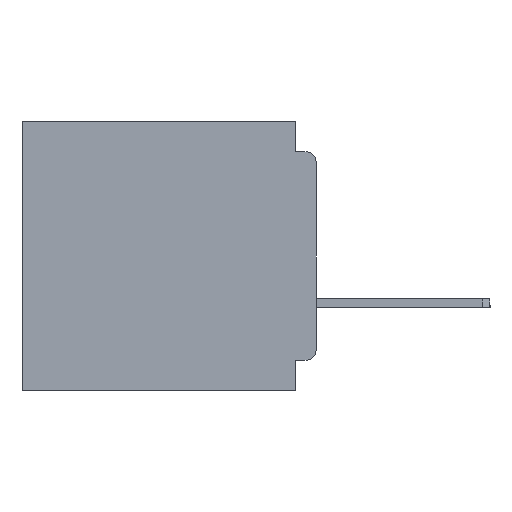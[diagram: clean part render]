
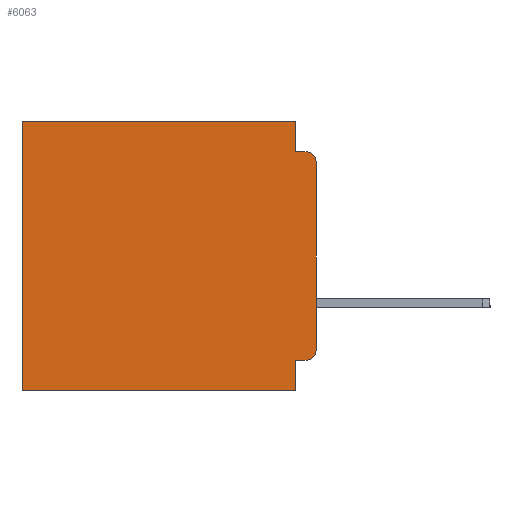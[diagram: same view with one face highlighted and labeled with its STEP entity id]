
A CAD part, left-side view. The second image highlights one B-rep face of the part: STEP entity #6063.
In plain terms, the highlighted planar face has unit normal (-1, 0, 0).
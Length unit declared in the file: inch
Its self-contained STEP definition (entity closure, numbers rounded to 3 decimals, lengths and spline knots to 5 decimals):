
#870 = CARTESIAN_POINT ( 'NONE',  ( 0.3, 0.031, -0.355 ) ) ;
#1079 = DIRECTION ( 'NONE',  ( 0., 0., -1. ) ) ;
#2589 = CARTESIAN_POINT ( 'NONE',  ( 0.3, 0.437, -0.4 ) ) ;
#3789 = VECTOR ( 'NONE', #7308, 39.37008 ) ;
#5596 = ORIENTED_EDGE ( 'NONE', *, *, #23079, .F. ) ;
#6063 = ADVANCED_FACE ( 'NONE', ( #39883 ), #53114, .F. ) ;
#6574 = VERTEX_POINT ( 'NONE', #17588 ) ;
#6836 = EDGE_LOOP ( 'NONE', ( #43528, #13128, #16899, #50039, #42352, #41228, #26954, #5596, #57168, #17152 ) ) ;
#7308 = DIRECTION ( 'NONE',  ( 0., -1., 0. ) ) ;
#7414 = CARTESIAN_POINT ( 'NONE',  ( 0.3, 0.031, 0. ) ) ;
#7686 = VECTOR ( 'NONE', #46446, 39.37008 ) ;
#8356 = EDGE_CURVE ( 'NONE', #29767, #29869, #30248, .T. ) ;
#10212 = CARTESIAN_POINT ( 'NONE',  ( 0.3, 0., 0. ) ) ;
#12451 = LINE ( 'NONE', #47709, #46542 ) ;
#12472 = CIRCLE ( 'NONE', #53079, 0.015 ) ;
#12743 = LINE ( 'NONE', #10212, #23214 ) ;
#13128 = ORIENTED_EDGE ( 'NONE', *, *, #23409, .T. ) ;
#13582 = CARTESIAN_POINT ( 'NONE',  ( 0.3, 0.015, -0.355 ) ) ;
#13831 = VERTEX_POINT ( 'NONE', #2589 ) ;
#14604 = DIRECTION ( 'NONE',  ( 0., 0., -1. ) ) ;
#15344 = CARTESIAN_POINT ( 'NONE',  ( 0.3, 0., -0.355 ) ) ;
#15393 = CARTESIAN_POINT ( 'NONE',  ( 0.3, 0.015, -0.045 ) ) ;
#15632 = VERTEX_POINT ( 'NONE', #38677 ) ;
#16899 = ORIENTED_EDGE ( 'NONE', *, *, #46309, .F. ) ;
#17152 = ORIENTED_EDGE ( 'NONE', *, *, #24739, .T. ) ;
#17314 = CARTESIAN_POINT ( 'NONE',  ( 0.3, 0., -0.06 ) ) ;
#17588 = CARTESIAN_POINT ( 'NONE',  ( 0.3, 0.031, -0.045 ) ) ;
#18169 = LINE ( 'NONE', #15344, #7686 ) ;
#18405 = VECTOR ( 'NONE', #23178, 39.37008 ) ;
#20305 = CARTESIAN_POINT ( 'NONE',  ( 0.3, 0.015, -0.34 ) ) ;
#20718 = VERTEX_POINT ( 'NONE', #15393 ) ;
#23079 = EDGE_CURVE ( 'NONE', #51175, #15632, #42421, .T. ) ;
#23178 = DIRECTION ( 'NONE',  ( 0., 0., -1. ) ) ;
#23214 = VECTOR ( 'NONE', #28918, 39.37008 ) ;
#23409 = EDGE_CURVE ( 'NONE', #29767, #20718, #12472, .T. ) ;
#23652 = CARTESIAN_POINT ( 'NONE',  ( 0.3, 0., -0.4 ) ) ;
#24739 = EDGE_CURVE ( 'NONE', #35865, #29869, #43616, .T. ) ;
#24775 = DIRECTION ( 'NONE',  ( 0., 0., -1. ) ) ;
#24956 = CARTESIAN_POINT ( 'NONE',  ( 0.3, 0.031, -0.4 ) ) ;
#26872 = VECTOR ( 'NONE', #50390, 39.37008 ) ;
#26954 = ORIENTED_EDGE ( 'NONE', *, *, #46728, .F. ) ;
#27821 = DIRECTION ( 'NONE',  ( -1., 0., 0. ) ) ;
#28078 = AXIS2_PLACEMENT_3D ( 'NONE', #30869, #57437, #31056 ) ;
#28918 = DIRECTION ( 'NONE',  ( 0., 1., 0. ) ) ;
#29539 = CARTESIAN_POINT ( 'NONE',  ( 0.3, 0., -0.045 ) ) ;
#29767 = VERTEX_POINT ( 'NONE', #17314 ) ;
#29869 = VERTEX_POINT ( 'NONE', #53360 ) ;
#30248 = LINE ( 'NONE', #54134, #18405 ) ;
#30644 = VECTOR ( 'NONE', #55897, 39.37008 ) ;
#30869 = CARTESIAN_POINT ( 'NONE',  ( 0.3, 0., -0.4 ) ) ;
#31056 = DIRECTION ( 'NONE',  ( 0., 0., -1. ) ) ;
#34215 = LINE ( 'NONE', #41252, #54950 ) ;
#35865 = VERTEX_POINT ( 'NONE', #13582 ) ;
#38677 = CARTESIAN_POINT ( 'NONE',  ( 0.3, 0.031, -0.4 ) ) ;
#38699 = LINE ( 'NONE', #23652, #26872 ) ;
#39642 = EDGE_CURVE ( 'NONE', #40361, #54009, #12743, .T. ) ;
#39883 = FACE_OUTER_BOUND ( 'NONE', #6836, .T. ) ;
#40361 = VERTEX_POINT ( 'NONE', #7414 ) ;
#41228 = ORIENTED_EDGE ( 'NONE', *, *, #43047, .T. ) ;
#41252 = CARTESIAN_POINT ( 'NONE',  ( 0.3, 0.437, -0.4 ) ) ;
#42352 = ORIENTED_EDGE ( 'NONE', *, *, #39642, .T. ) ;
#42421 = LINE ( 'NONE', #24956, #30644 ) ;
#43047 = EDGE_CURVE ( 'NONE', #54009, #13831, #34215, .T. ) ;
#43528 = ORIENTED_EDGE ( 'NONE', *, *, #8356, .F. ) ;
#43616 = CIRCLE ( 'NONE', #46518, 0.015 ) ;
#44488 = EDGE_CURVE ( 'NONE', #40361, #6574, #12451, .T. ) ;
#46309 = EDGE_CURVE ( 'NONE', #6574, #20718, #51117, .T. ) ;
#46446 = DIRECTION ( 'NONE',  ( 0., 1., 0. ) ) ;
#46518 = AXIS2_PLACEMENT_3D ( 'NONE', #20305, #51313, #24775 ) ;
#46542 = VECTOR ( 'NONE', #51940, 39.37008 ) ;
#46728 = EDGE_CURVE ( 'NONE', #15632, #13831, #38699, .T. ) ;
#47709 = CARTESIAN_POINT ( 'NONE',  ( 0.3, 0.031, 0. ) ) ;
#49612 = CARTESIAN_POINT ( 'NONE',  ( 0.3, 0.437, 0. ) ) ;
#50039 = ORIENTED_EDGE ( 'NONE', *, *, #44488, .F. ) ;
#50390 = DIRECTION ( 'NONE',  ( 0., 1., 0. ) ) ;
#51117 = LINE ( 'NONE', #29539, #3789 ) ;
#51175 = VERTEX_POINT ( 'NONE', #870 ) ;
#51313 = DIRECTION ( 'NONE',  ( -1., 0., 0. ) ) ;
#51940 = DIRECTION ( 'NONE',  ( 0., 0., -1. ) ) ;
#53079 = AXIS2_PLACEMENT_3D ( 'NONE', #54358, #27821, #1079 ) ;
#53114 = PLANE ( 'NONE',  #28078 ) ;
#53360 = CARTESIAN_POINT ( 'NONE',  ( 0.3, 0., -0.34 ) ) ;
#54009 = VERTEX_POINT ( 'NONE', #49612 ) ;
#54134 = CARTESIAN_POINT ( 'NONE',  ( 0.3, 0., -0.4 ) ) ;
#54358 = CARTESIAN_POINT ( 'NONE',  ( 0.3, 0.015, -0.06 ) ) ;
#54950 = VECTOR ( 'NONE', #14604, 39.37008 ) ;
#55897 = DIRECTION ( 'NONE',  ( 0., 0., -1. ) ) ;
#56164 = EDGE_CURVE ( 'NONE', #35865, #51175, #18169, .T. ) ;
#57168 = ORIENTED_EDGE ( 'NONE', *, *, #56164, .F. ) ;
#57437 = DIRECTION ( 'NONE',  ( 1., 0., 0. ) ) ;
